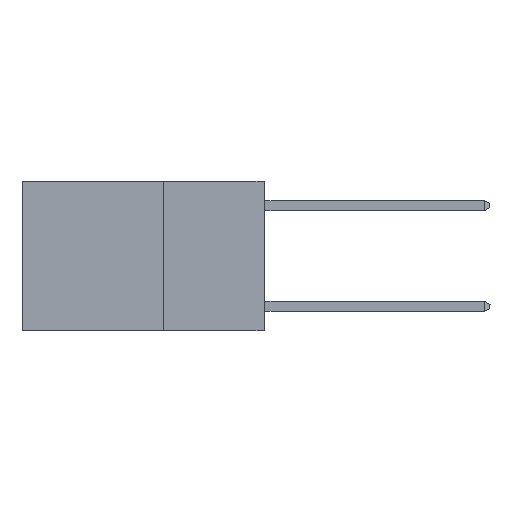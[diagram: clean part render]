
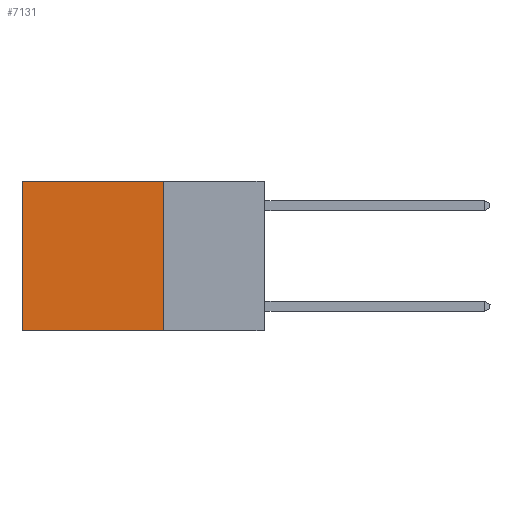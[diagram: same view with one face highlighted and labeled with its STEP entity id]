
A CAD part, left-side view. The second image highlights one B-rep face of the part: STEP entity #7131.
In plain terms, the highlighted planar face has unit normal (-1, 0, 0).
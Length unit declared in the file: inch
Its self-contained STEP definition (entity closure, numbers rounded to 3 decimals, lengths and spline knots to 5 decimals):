
#437 = ORIENTED_EDGE ( 'NONE', *, *, #5068, .T. ) ;
#1311 = DIRECTION ( 'NONE',  ( 0., 1., 0. ) ) ;
#1818 = VERTEX_POINT ( 'NONE', #10889 ) ;
#2930 = CARTESIAN_POINT ( 'NONE',  ( 0.2625, 0.25, -0.37 ) ) ;
#3341 = LINE ( 'NONE', #15051, #9303 ) ;
#3717 = PLANE ( 'NONE',  #5088 ) ;
#3805 = CARTESIAN_POINT ( 'NONE',  ( 0.2625, 0.6, 0. ) ) ;
#3877 = CARTESIAN_POINT ( 'NONE',  ( 0.2625, 0.25, 0. ) ) ;
#4643 = VERTEX_POINT ( 'NONE', #11840 ) ;
#4878 = EDGE_CURVE ( 'NONE', #4643, #1818, #12985, .T. ) ;
#5015 = EDGE_CURVE ( 'NONE', #6146, #1818, #3341, .T. ) ;
#5068 = EDGE_CURVE ( 'NONE', #6096, #4643, #5674, .T. ) ;
#5088 = AXIS2_PLACEMENT_3D ( 'NONE', #14612, #12086, #5101 ) ;
#5101 = DIRECTION ( 'NONE',  ( 0., 0., -1. ) ) ;
#5465 = VECTOR ( 'NONE', #17678, 39.37008 ) ;
#5674 = LINE ( 'NONE', #15103, #16196 ) ;
#6096 = VERTEX_POINT ( 'NONE', #17519 ) ;
#6146 = VERTEX_POINT ( 'NONE', #2930 ) ;
#6506 = DIRECTION ( 'NONE',  ( 0., 0., -1. ) ) ;
#6513 = ORIENTED_EDGE ( 'NONE', *, *, #7795, .F. ) ;
#6546 = ORIENTED_EDGE ( 'NONE', *, *, #4878, .T. ) ;
#7131 = ADVANCED_FACE ( 'NONE', ( #13212 ), #3717, .F. ) ;
#7795 = EDGE_CURVE ( 'NONE', #6096, #6146, #15429, .T. ) ;
#9303 = VECTOR ( 'NONE', #1311, 39.37008 ) ;
#9575 = DIRECTION ( 'NONE',  ( 0., 1., 0. ) ) ;
#10889 = CARTESIAN_POINT ( 'NONE',  ( 0.2625, 0.6, -0.37 ) ) ;
#11840 = CARTESIAN_POINT ( 'NONE',  ( 0.2625, 0.6, 0. ) ) ;
#12086 = DIRECTION ( 'NONE',  ( 1., 0., 0. ) ) ;
#12662 = EDGE_LOOP ( 'NONE', ( #6546, #16598, #6513, #437 ) ) ;
#12985 = LINE ( 'NONE', #3805, #5465 ) ;
#13212 = FACE_OUTER_BOUND ( 'NONE', #12662, .T. ) ;
#14612 = CARTESIAN_POINT ( 'NONE',  ( 0.2625, 0.25, 0. ) ) ;
#14993 = VECTOR ( 'NONE', #6506, 39.37008 ) ;
#15051 = CARTESIAN_POINT ( 'NONE',  ( 0.2625, 0.25, -0.37 ) ) ;
#15103 = CARTESIAN_POINT ( 'NONE',  ( 0.2625, 0.25, 0. ) ) ;
#15429 = LINE ( 'NONE', #3877, #14993 ) ;
#16196 = VECTOR ( 'NONE', #9575, 39.37008 ) ;
#16598 = ORIENTED_EDGE ( 'NONE', *, *, #5015, .F. ) ;
#17519 = CARTESIAN_POINT ( 'NONE',  ( 0.2625, 0.25, 0. ) ) ;
#17678 = DIRECTION ( 'NONE',  ( 0., 0., -1. ) ) ;
